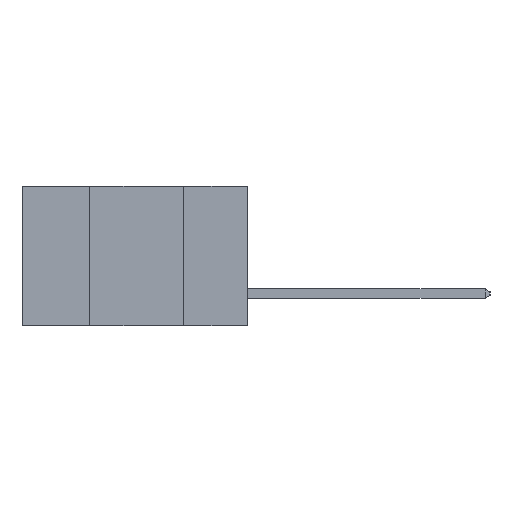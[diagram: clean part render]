
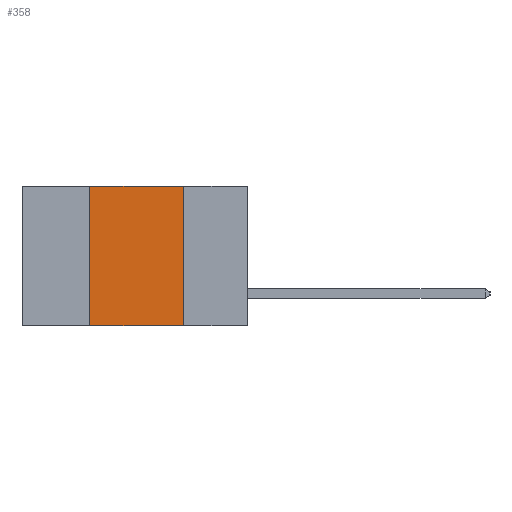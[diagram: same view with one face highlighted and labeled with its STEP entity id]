
A CAD part, left-side view. The second image highlights one B-rep face of the part: STEP entity #358.
In plain terms, the highlighted planar face has unit normal (-1, 0, 0).
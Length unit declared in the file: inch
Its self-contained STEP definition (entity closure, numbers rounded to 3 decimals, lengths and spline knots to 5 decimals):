
#358 = ADVANCED_FACE ( 'NONE', ( #1831 ), #8466, .F. ) ;
#916 = AXIS2_PLACEMENT_3D ( 'NONE', #13237, #12187, #12080 ) ;
#1268 = VERTEX_POINT ( 'NONE', #11391 ) ;
#1831 = FACE_OUTER_BOUND ( 'NONE', #8604, .T. ) ;
#2027 = LINE ( 'NONE', #5799, #12873 ) ;
#3041 = CARTESIAN_POINT ( 'NONE',  ( 0., 0.42, 0. ) ) ;
#3448 = ORIENTED_EDGE ( 'NONE', *, *, #4192, .F. ) ;
#3490 = VERTEX_POINT ( 'NONE', #8360 ) ;
#3671 = EDGE_CURVE ( 'NONE', #3490, #4358, #11265, .T. ) ;
#3743 = CARTESIAN_POINT ( 'NONE',  ( 0., 0.17, 0. ) ) ;
#3918 = DIRECTION ( 'NONE',  ( 0., -1., 0. ) ) ;
#4192 = EDGE_CURVE ( 'NONE', #1268, #13454, #12892, .T. ) ;
#4358 = VERTEX_POINT ( 'NONE', #8938 ) ;
#4673 = VECTOR ( 'NONE', #11663, 39.37008 ) ;
#5014 = EDGE_CURVE ( 'NONE', #1268, #4358, #2027, .T. ) ;
#5395 = VECTOR ( 'NONE', #7019, 39.37008 ) ;
#5536 = ORIENTED_EDGE ( 'NONE', *, *, #9559, .F. ) ;
#5799 = CARTESIAN_POINT ( 'NONE',  ( 0., 0.6, -0.37 ) ) ;
#7019 = DIRECTION ( 'NONE',  ( 0., 0., -1. ) ) ;
#7183 = CARTESIAN_POINT ( 'NONE',  ( 0., 0.6, 0. ) ) ;
#8360 = CARTESIAN_POINT ( 'NONE',  ( 0., 0.17, 0. ) ) ;
#8466 = PLANE ( 'NONE',  #916 ) ;
#8604 = EDGE_LOOP ( 'NONE', ( #9753, #5536, #3448, #11072 ) ) ;
#8938 = CARTESIAN_POINT ( 'NONE',  ( 0., 0.17, -0.37 ) ) ;
#9559 = EDGE_CURVE ( 'NONE', #13454, #3490, #9811, .T. ) ;
#9753 = ORIENTED_EDGE ( 'NONE', *, *, #3671, .F. ) ;
#9811 = LINE ( 'NONE', #7183, #12076 ) ;
#11072 = ORIENTED_EDGE ( 'NONE', *, *, #5014, .T. ) ;
#11265 = LINE ( 'NONE', #3743, #5395 ) ;
#11391 = CARTESIAN_POINT ( 'NONE',  ( 0., 0.42, -0.37 ) ) ;
#11663 = DIRECTION ( 'NONE',  ( 0., 0., 1. ) ) ;
#11784 = CARTESIAN_POINT ( 'NONE',  ( 0., 0.42, 0. ) ) ;
#12076 = VECTOR ( 'NONE', #3918, 39.37008 ) ;
#12080 = DIRECTION ( 'NONE',  ( 0., 0., -1. ) ) ;
#12187 = DIRECTION ( 'NONE',  ( 1., 0., 0. ) ) ;
#12873 = VECTOR ( 'NONE', #13173, 39.37008 ) ;
#12892 = LINE ( 'NONE', #3041, #4673 ) ;
#13173 = DIRECTION ( 'NONE',  ( 0., -1., 0. ) ) ;
#13237 = CARTESIAN_POINT ( 'NONE',  ( 0., 0.6, 0. ) ) ;
#13454 = VERTEX_POINT ( 'NONE', #11784 ) ;
